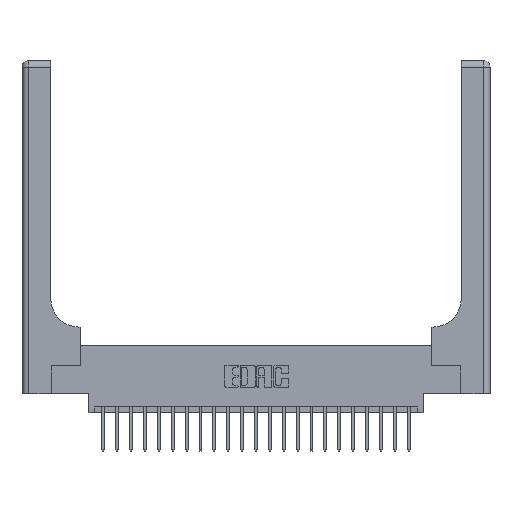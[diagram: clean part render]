
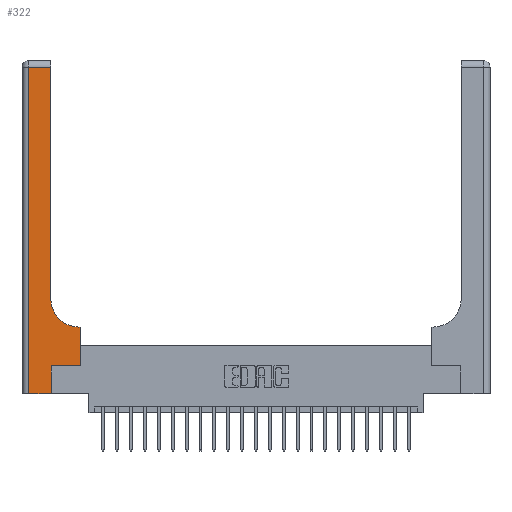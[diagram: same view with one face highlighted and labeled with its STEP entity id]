
A CAD part, top view. The second image highlights one B-rep face of the part: STEP entity #322.
In plain terms, the highlighted planar face has unit normal (0, 0, 1).
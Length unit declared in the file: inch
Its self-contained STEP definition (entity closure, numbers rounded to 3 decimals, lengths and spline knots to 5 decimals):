
#223 = VERTEX_POINT ( 'NONE', #13014 ) ;
#240 = EDGE_CURVE ( 'NONE', #20826, #223, #11159, .T. ) ;
#322 = ADVANCED_FACE ( 'NONE', ( #2153 ), #498, .F. ) ;
#498 = PLANE ( 'NONE',  #1716 ) ;
#621 = LINE ( 'NONE', #22238, #2627 ) ;
#850 = DIRECTION ( 'NONE',  ( 0., -1., 0. ) ) ;
#860 = ORIENTED_EDGE ( 'NONE', *, *, #18436, .T. ) ;
#1299 = CARTESIAN_POINT ( 'NONE',  ( 0.26, 2.94, 0.37 ) ) ;
#1609 = EDGE_LOOP ( 'NONE', ( #16723, #18489, #4761, #860, #21411, #5158, #16358, #14597, #8648 ) ) ;
#1702 = VERTEX_POINT ( 'NONE', #1299 ) ;
#1716 = AXIS2_PLACEMENT_3D ( 'NONE', #22003, #5829, #7697 ) ;
#2044 = DIRECTION ( 'NONE',  ( 0., 0., -1. ) ) ;
#2153 = FACE_OUTER_BOUND ( 'NONE', #1609, .T. ) ;
#2627 = VECTOR ( 'NONE', #850, 39.37008 ) ;
#2755 = DIRECTION ( 'NONE',  ( 0., 1., 0. ) ) ;
#3398 = LINE ( 'NONE', #3877, #3490 ) ;
#3460 = VECTOR ( 'NONE', #19321, 39.37008 ) ;
#3490 = VECTOR ( 'NONE', #11079, 39.37008 ) ;
#3553 = EDGE_CURVE ( 'NONE', #223, #1702, #5074, .T. ) ;
#3877 = CARTESIAN_POINT ( 'NONE',  ( 0., 0., 0.37 ) ) ;
#4288 = CARTESIAN_POINT ( 'NONE',  ( 0.265, 0., 0.37 ) ) ;
#4315 = EDGE_CURVE ( 'NONE', #17889, #22674, #16354, .T. ) ;
#4496 = CARTESIAN_POINT ( 'NONE',  ( 0.51, 0.6, 0.37 ) ) ;
#4638 = DIRECTION ( 'NONE',  ( -1., 0., 0. ) ) ;
#4761 = ORIENTED_EDGE ( 'NONE', *, *, #13659, .T. ) ;
#5074 = LINE ( 'NONE', #9075, #22950 ) ;
#5158 = ORIENTED_EDGE ( 'NONE', *, *, #4315, .T. ) ;
#5612 = CARTESIAN_POINT ( 'NONE',  ( 0.265, 0.25, 0.37 ) ) ;
#5653 = DIRECTION ( 'NONE',  ( -1., 0., 0. ) ) ;
#5829 = DIRECTION ( 'NONE',  ( 0., 0., -1. ) ) ;
#6825 = CARTESIAN_POINT ( 'NONE',  ( 0.528, 0.25, 0.37 ) ) ;
#7383 = DIRECTION ( 'NONE',  ( 1., 0., 0. ) ) ;
#7697 = DIRECTION ( 'NONE',  ( -1., 0., 0. ) ) ;
#7818 = LINE ( 'NONE', #17136, #12087 ) ;
#8648 = ORIENTED_EDGE ( 'NONE', *, *, #240, .T. ) ;
#9006 = CARTESIAN_POINT ( 'NONE',  ( 0.06, 0., 0.37 ) ) ;
#9075 = CARTESIAN_POINT ( 'NONE',  ( 0.26, 3., 0.37 ) ) ;
#10637 = VECTOR ( 'NONE', #22128, 39.37008 ) ;
#11079 = DIRECTION ( 'NONE',  ( 1., 0., 0. ) ) ;
#11159 = CIRCLE ( 'NONE', #21717, 0.25 ) ;
#11354 = CARTESIAN_POINT ( 'NONE',  ( 0.51, 0.85, 0.37 ) ) ;
#11368 = CARTESIAN_POINT ( 'NONE',  ( 0.265, 0.25, 0.37 ) ) ;
#11466 = VERTEX_POINT ( 'NONE', #18715 ) ;
#11674 = CARTESIAN_POINT ( 'NONE',  ( 0.528, 0.6, 0.37 ) ) ;
#12087 = VECTOR ( 'NONE', #4638, 39.37008 ) ;
#13014 = CARTESIAN_POINT ( 'NONE',  ( 0.26, 0.85, 0.37 ) ) ;
#13399 = VECTOR ( 'NONE', #7383, 39.37008 ) ;
#13659 = EDGE_CURVE ( 'NONE', #11466, #23049, #621, .T. ) ;
#13817 = VERTEX_POINT ( 'NONE', #11674 ) ;
#14333 = VECTOR ( 'NONE', #5653, 39.37008 ) ;
#14425 = LINE ( 'NONE', #6825, #3460 ) ;
#14597 = ORIENTED_EDGE ( 'NONE', *, *, #23149, .T. ) ;
#14627 = LINE ( 'NONE', #21825, #14333 ) ;
#15117 = CARTESIAN_POINT ( 'NONE',  ( 0.265, 0., 0.37 ) ) ;
#15651 = VERTEX_POINT ( 'NONE', #15117 ) ;
#16344 = EDGE_CURVE ( 'NONE', #15651, #17889, #18333, .T. ) ;
#16354 = LINE ( 'NONE', #5612, #13399 ) ;
#16358 = ORIENTED_EDGE ( 'NONE', *, *, #17473, .T. ) ;
#16723 = ORIENTED_EDGE ( 'NONE', *, *, #3553, .T. ) ;
#17136 = CARTESIAN_POINT ( 'NONE',  ( 0.26, 0.6, 0.37 ) ) ;
#17473 = EDGE_CURVE ( 'NONE', #22674, #13817, #14425, .T. ) ;
#17889 = VERTEX_POINT ( 'NONE', #11368 ) ;
#18333 = LINE ( 'NONE', #4288, #10637 ) ;
#18436 = EDGE_CURVE ( 'NONE', #23049, #15651, #3398, .T. ) ;
#18489 = ORIENTED_EDGE ( 'NONE', *, *, #21476, .T. ) ;
#18715 = CARTESIAN_POINT ( 'NONE',  ( 0.06, 2.94, 0.37 ) ) ;
#19321 = DIRECTION ( 'NONE',  ( 0., 1., 0. ) ) ;
#20826 = VERTEX_POINT ( 'NONE', #4496 ) ;
#21411 = ORIENTED_EDGE ( 'NONE', *, *, #16344, .T. ) ;
#21476 = EDGE_CURVE ( 'NONE', #1702, #11466, #14627, .T. ) ;
#21717 = AXIS2_PLACEMENT_3D ( 'NONE', #11354, #2044, #22217 ) ;
#21825 = CARTESIAN_POINT ( 'NONE',  ( 0., 2.94, 0.37 ) ) ;
#22003 = CARTESIAN_POINT ( 'NONE',  ( 0., 3., 0.37 ) ) ;
#22128 = DIRECTION ( 'NONE',  ( 0., 1., 0. ) ) ;
#22217 = DIRECTION ( 'NONE',  ( 1., 0., 0. ) ) ;
#22238 = CARTESIAN_POINT ( 'NONE',  ( 0.06, 3., 0.37 ) ) ;
#22674 = VERTEX_POINT ( 'NONE', #22731 ) ;
#22731 = CARTESIAN_POINT ( 'NONE',  ( 0.528, 0.25, 0.37 ) ) ;
#22950 = VECTOR ( 'NONE', #2755, 39.37008 ) ;
#23049 = VERTEX_POINT ( 'NONE', #9006 ) ;
#23149 = EDGE_CURVE ( 'NONE', #13817, #20826, #7818, .T. ) ;
